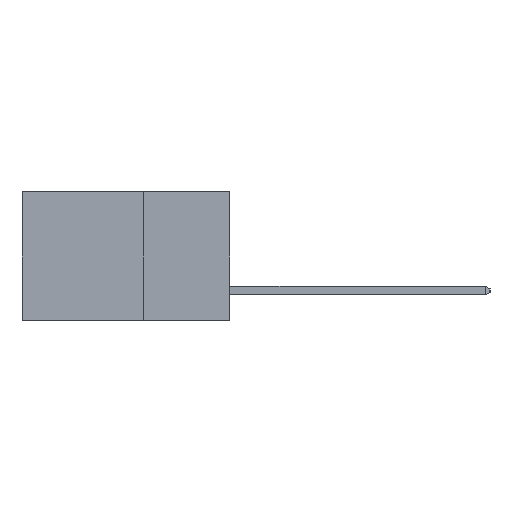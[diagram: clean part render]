
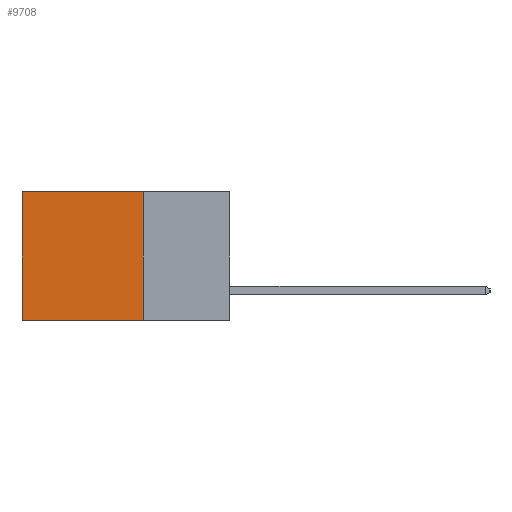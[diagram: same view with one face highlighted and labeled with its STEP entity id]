
A CAD part, left-side view. The second image highlights one B-rep face of the part: STEP entity #9708.
In plain terms, the highlighted planar face has unit normal (-1, 0, 0).
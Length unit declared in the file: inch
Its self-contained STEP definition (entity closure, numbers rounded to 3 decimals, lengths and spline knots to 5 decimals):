
#42 = AXIS2_PLACEMENT_3D ( 'NONE', #5687, #429, #6450 ) ;
#58 = ORIENTED_EDGE ( 'NONE', *, *, #9124, .F. ) ;
#63 = EDGE_CURVE ( 'NONE', #609, #1772, #6961, .T. ) ;
#161 = CARTESIAN_POINT ( 'NONE',  ( 0.2615, 0.25, -0.37 ) ) ;
#424 = VECTOR ( 'NONE', #2915, 39.37008 ) ;
#429 = DIRECTION ( 'NONE',  ( 1., 0., 0. ) ) ;
#609 = VERTEX_POINT ( 'NONE', #8900 ) ;
#1176 = DIRECTION ( 'NONE',  ( 0., 0., -1. ) ) ;
#1772 = VERTEX_POINT ( 'NONE', #3130 ) ;
#2045 = CARTESIAN_POINT ( 'NONE',  ( 0.2615, 0.25, -0.37 ) ) ;
#2217 = CARTESIAN_POINT ( 'NONE',  ( 0.2615, 0.6, -0.37 ) ) ;
#2915 = DIRECTION ( 'NONE',  ( 0., 0., -1. ) ) ;
#2960 = ORIENTED_EDGE ( 'NONE', *, *, #9137, .F. ) ;
#3023 = CARTESIAN_POINT ( 'NONE',  ( 0.2615, 0.25, -0.37 ) ) ;
#3040 = CARTESIAN_POINT ( 'NONE',  ( 0.2615, 0.25, 0. ) ) ;
#3130 = CARTESIAN_POINT ( 'NONE',  ( 0.2615, 0.6, -0.37 ) ) ;
#3560 = VERTEX_POINT ( 'NONE', #10277 ) ;
#3915 = DIRECTION ( 'NONE',  ( 0., 1., 0. ) ) ;
#4066 = PLANE ( 'NONE',  #42 ) ;
#4492 = LINE ( 'NONE', #3040, #6553 ) ;
#4520 = VECTOR ( 'NONE', #1176, 39.37008 ) ;
#4753 = DIRECTION ( 'NONE',  ( 0., 1., 0. ) ) ;
#4778 = LINE ( 'NONE', #3023, #8378 ) ;
#4779 = ORIENTED_EDGE ( 'NONE', *, *, #10238, .T. ) ;
#5687 = CARTESIAN_POINT ( 'NONE',  ( 0.2615, 0.25, -0.37 ) ) ;
#5744 = FACE_OUTER_BOUND ( 'NONE', #6579, .T. ) ;
#6450 = DIRECTION ( 'NONE',  ( 0., 0., -1. ) ) ;
#6553 = VECTOR ( 'NONE', #4753, 39.37008 ) ;
#6578 = LINE ( 'NONE', #2045, #4520 ) ;
#6579 = EDGE_LOOP ( 'NONE', ( #8074, #2960, #58, #4779 ) ) ;
#6961 = LINE ( 'NONE', #2217, #424 ) ;
#7557 = VERTEX_POINT ( 'NONE', #161 ) ;
#8074 = ORIENTED_EDGE ( 'NONE', *, *, #63, .T. ) ;
#8378 = VECTOR ( 'NONE', #3915, 39.37008 ) ;
#8900 = CARTESIAN_POINT ( 'NONE',  ( 0.2615, 0.6, 0. ) ) ;
#9124 = EDGE_CURVE ( 'NONE', #3560, #7557, #6578, .T. ) ;
#9137 = EDGE_CURVE ( 'NONE', #7557, #1772, #4778, .T. ) ;
#9708 = ADVANCED_FACE ( 'NONE', ( #5744 ), #4066, .F. ) ;
#10238 = EDGE_CURVE ( 'NONE', #3560, #609, #4492, .T. ) ;
#10277 = CARTESIAN_POINT ( 'NONE',  ( 0.2615, 0.25, 0. ) ) ;
